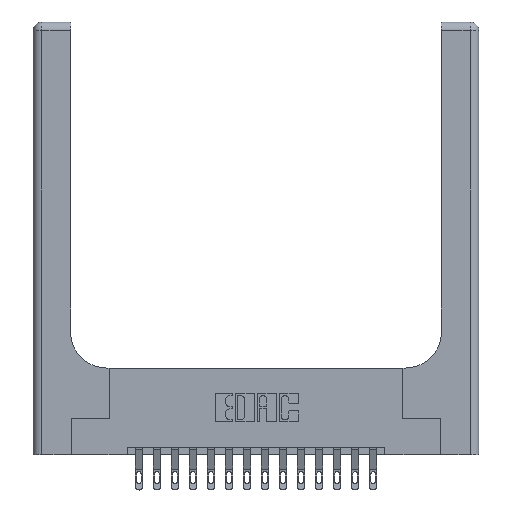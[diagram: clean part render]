
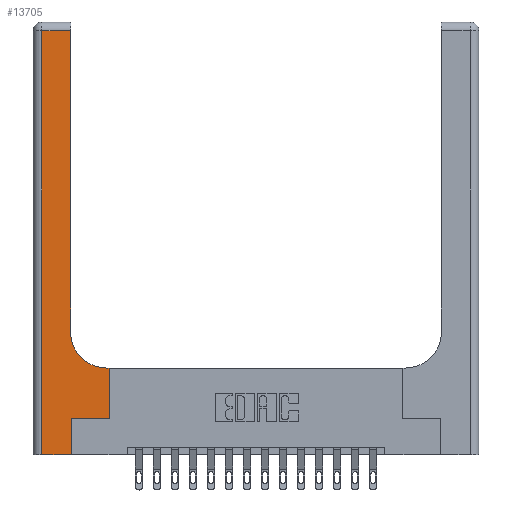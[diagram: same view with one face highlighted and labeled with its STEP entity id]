
A CAD part, top view. The second image highlights one B-rep face of the part: STEP entity #13705.
In plain terms, the highlighted planar face has unit normal (0, 0, 1).
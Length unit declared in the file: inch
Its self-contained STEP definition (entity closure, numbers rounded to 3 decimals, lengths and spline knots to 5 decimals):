
#139 = VERTEX_POINT ( 'NONE', #14720 ) ;
#418 = AXIS2_PLACEMENT_3D ( 'NONE', #1252, #15431, #9796 ) ;
#496 = LINE ( 'NONE', #17112, #10287 ) ;
#528 = LINE ( 'NONE', #10677, #9659 ) ;
#719 = LINE ( 'NONE', #11113, #3596 ) ;
#1252 = CARTESIAN_POINT ( 'NONE',  ( 0., 3., 0.37 ) ) ;
#1653 = CARTESIAN_POINT ( 'NONE',  ( 0.528, 0.25, 0.37 ) ) ;
#2070 = LINE ( 'NONE', #12285, #6306 ) ;
#2730 = EDGE_CURVE ( 'NONE', #5207, #14029, #496, .T. ) ;
#2878 = EDGE_CURVE ( 'NONE', #10944, #5207, #8509, .T. ) ;
#2998 = EDGE_CURVE ( 'NONE', #18029, #139, #719, .T. ) ;
#3122 = DIRECTION ( 'NONE',  ( -1., 0., 0. ) ) ;
#3543 = DIRECTION ( 'NONE',  ( 0., 0., -1. ) ) ;
#3596 = VECTOR ( 'NONE', #18161, 39.37008 ) ;
#3773 = DIRECTION ( 'NONE',  ( -1., 0., 0. ) ) ;
#4451 = DIRECTION ( 'NONE',  ( 0., 1., 0. ) ) ;
#4532 = LINE ( 'NONE', #12668, #17428 ) ;
#4610 = VERTEX_POINT ( 'NONE', #16440 ) ;
#4944 = CARTESIAN_POINT ( 'NONE',  ( 0.06, 0., 0.37 ) ) ;
#5078 = VECTOR ( 'NONE', #7392, 39.37008 ) ;
#5207 = VERTEX_POINT ( 'NONE', #13762 ) ;
#6306 = VECTOR ( 'NONE', #3773, 39.37008 ) ;
#6637 = ORIENTED_EDGE ( 'NONE', *, *, #17284, .T. ) ;
#6716 = ORIENTED_EDGE ( 'NONE', *, *, #10745, .T. ) ;
#6760 = CARTESIAN_POINT ( 'NONE',  ( 0., 0., 0.37 ) ) ;
#7392 = DIRECTION ( 'NONE',  ( 1., 0., 0. ) ) ;
#7418 = CARTESIAN_POINT ( 'NONE',  ( 0.528, 0.25, 0.37 ) ) ;
#7685 = EDGE_LOOP ( 'NONE', ( #14496, #13888, #9903, #6716, #16542, #6637, #10840, #13973, #9147 ) ) ;
#7901 = CARTESIAN_POINT ( 'NONE',  ( 0.51, 0.85, 0.37 ) ) ;
#8011 = EDGE_CURVE ( 'NONE', #14029, #4610, #4532, .T. ) ;
#8251 = EDGE_CURVE ( 'NONE', #4610, #13353, #528, .T. ) ;
#8459 = EDGE_CURVE ( 'NONE', #13895, #16082, #11851, .T. ) ;
#8494 = CARTESIAN_POINT ( 'NONE',  ( 0.265, 0., 0.37 ) ) ;
#8509 = CIRCLE ( 'NONE', #12706, 0.25 ) ;
#8593 = EDGE_CURVE ( 'NONE', #16082, #10944, #2070, .T. ) ;
#8595 = DIRECTION ( 'NONE',  ( 0., 1., 0. ) ) ;
#8810 = CARTESIAN_POINT ( 'NONE',  ( 0.265, 0.25, 0.37 ) ) ;
#8920 = VECTOR ( 'NONE', #12415, 39.37008 ) ;
#9147 = ORIENTED_EDGE ( 'NONE', *, *, #2878, .T. ) ;
#9377 = DIRECTION ( 'NONE',  ( 0., -1., 0. ) ) ;
#9659 = VECTOR ( 'NONE', #9377, 39.37008 ) ;
#9796 = DIRECTION ( 'NONE',  ( -1., 0., 0. ) ) ;
#9903 = ORIENTED_EDGE ( 'NONE', *, *, #8251, .T. ) ;
#10287 = VECTOR ( 'NONE', #8595, 39.37008 ) ;
#10677 = CARTESIAN_POINT ( 'NONE',  ( 0.06, 3., 0.37 ) ) ;
#10745 = EDGE_CURVE ( 'NONE', #13353, #18029, #12701, .T. ) ;
#10840 = ORIENTED_EDGE ( 'NONE', *, *, #8459, .T. ) ;
#10941 = FACE_OUTER_BOUND ( 'NONE', #7685, .T. ) ;
#10944 = VERTEX_POINT ( 'NONE', #16944 ) ;
#11113 = CARTESIAN_POINT ( 'NONE',  ( 0.265, 0., 0.37 ) ) ;
#11851 = LINE ( 'NONE', #1653, #15208 ) ;
#12181 = DIRECTION ( 'NONE',  ( 1., 0., 0. ) ) ;
#12285 = CARTESIAN_POINT ( 'NONE',  ( 0.26, 0.6, 0.37 ) ) ;
#12415 = DIRECTION ( 'NONE',  ( 1., 0., 0. ) ) ;
#12668 = CARTESIAN_POINT ( 'NONE',  ( 0., 2.94, 0.37 ) ) ;
#12701 = LINE ( 'NONE', #6760, #8920 ) ;
#12703 = PLANE ( 'NONE',  #418 ) ;
#12706 = AXIS2_PLACEMENT_3D ( 'NONE', #7901, #3543, #12181 ) ;
#13353 = VERTEX_POINT ( 'NONE', #4944 ) ;
#13616 = CARTESIAN_POINT ( 'NONE',  ( 0.26, 2.94, 0.37 ) ) ;
#13705 = ADVANCED_FACE ( 'NONE', ( #10941 ), #12703, .F. ) ;
#13762 = CARTESIAN_POINT ( 'NONE',  ( 0.26, 0.85, 0.37 ) ) ;
#13888 = ORIENTED_EDGE ( 'NONE', *, *, #8011, .T. ) ;
#13895 = VERTEX_POINT ( 'NONE', #7418 ) ;
#13973 = ORIENTED_EDGE ( 'NONE', *, *, #8593, .T. ) ;
#14029 = VERTEX_POINT ( 'NONE', #13616 ) ;
#14496 = ORIENTED_EDGE ( 'NONE', *, *, #2730, .T. ) ;
#14720 = CARTESIAN_POINT ( 'NONE',  ( 0.265, 0.25, 0.37 ) ) ;
#15208 = VECTOR ( 'NONE', #4451, 39.37008 ) ;
#15298 = LINE ( 'NONE', #8810, #5078 ) ;
#15431 = DIRECTION ( 'NONE',  ( 0., 0., -1. ) ) ;
#16082 = VERTEX_POINT ( 'NONE', #17243 ) ;
#16440 = CARTESIAN_POINT ( 'NONE',  ( 0.06, 2.94, 0.37 ) ) ;
#16542 = ORIENTED_EDGE ( 'NONE', *, *, #2998, .T. ) ;
#16944 = CARTESIAN_POINT ( 'NONE',  ( 0.51, 0.6, 0.37 ) ) ;
#17112 = CARTESIAN_POINT ( 'NONE',  ( 0.26, 3., 0.37 ) ) ;
#17243 = CARTESIAN_POINT ( 'NONE',  ( 0.528, 0.6, 0.37 ) ) ;
#17284 = EDGE_CURVE ( 'NONE', #139, #13895, #15298, .T. ) ;
#17428 = VECTOR ( 'NONE', #3122, 39.37008 ) ;
#18029 = VERTEX_POINT ( 'NONE', #8494 ) ;
#18161 = DIRECTION ( 'NONE',  ( 0., 1., 0. ) ) ;
